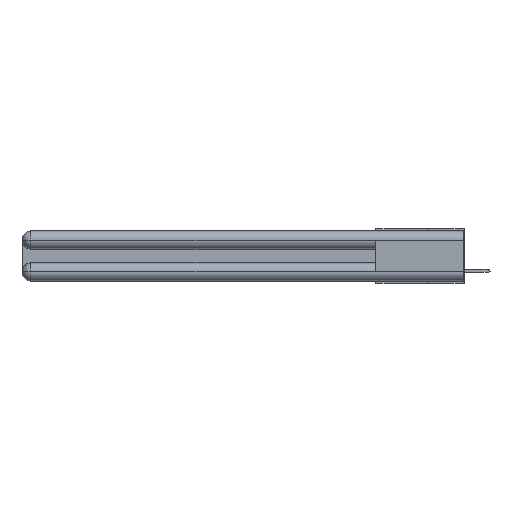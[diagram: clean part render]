
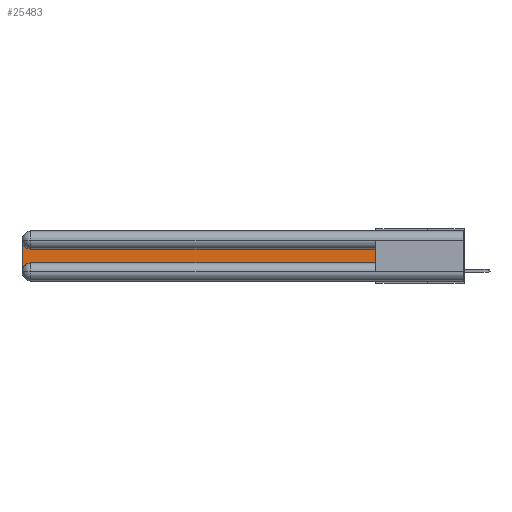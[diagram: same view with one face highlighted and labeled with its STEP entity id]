
A CAD part, left-side view. The second image highlights one B-rep face of the part: STEP entity #25483.
In plain terms, the highlighted planar face has unit normal (-1, 0, 0).
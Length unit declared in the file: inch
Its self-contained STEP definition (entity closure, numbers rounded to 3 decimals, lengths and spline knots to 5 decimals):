
#233 = FACE_OUTER_BOUND ( 'NONE', #18281, .T. ) ;
#754 = ORIENTED_EDGE ( 'NONE', *, *, #1114, .T. ) ;
#1114 = EDGE_CURVE ( 'NONE', #22305, #10074, #21309, .T. ) ;
#3070 = VERTEX_POINT ( 'NONE', #9788 ) ;
#3203 = CARTESIAN_POINT ( 'NONE',  ( 0.075, 3., -0.2175 ) ) ;
#3889 = CARTESIAN_POINT ( 'NONE',  ( 0.075, 0.6, -0.2175 ) ) ;
#4226 = CARTESIAN_POINT ( 'NONE',  ( 0.075, 2.94, -0.2175 ) ) ;
#4910 = ORIENTED_EDGE ( 'NONE', *, *, #23631, .T. ) ;
#5652 = VERTEX_POINT ( 'NONE', #27486 ) ;
#5672 = ORIENTED_EDGE ( 'NONE', *, *, #25782, .T. ) ;
#5896 = CARTESIAN_POINT ( 'NONE',  ( 0.075, 2.94, -0.1225 ) ) ;
#7028 = DIRECTION ( 'NONE',  ( 1., 0., 0. ) ) ;
#7158 = EDGE_CURVE ( 'NONE', #3070, #12762, #14640, .T. ) ;
#8700 = ORIENTED_EDGE ( 'NONE', *, *, #21315, .T. ) ;
#8756 = DIRECTION ( 'NONE',  ( 1., 0., 0. ) ) ;
#9788 = CARTESIAN_POINT ( 'NONE',  ( 0.075, 3., -0.2775 ) ) ;
#9934 = CIRCLE ( 'NONE', #12007, 0.06 ) ;
#10074 = VERTEX_POINT ( 'NONE', #5896 ) ;
#11092 = VECTOR ( 'NONE', #24347, 39.37008 ) ;
#11602 = VECTOR ( 'NONE', #26662, 39.37008 ) ;
#12007 = AXIS2_PLACEMENT_3D ( 'NONE', #19450, #8756, #13043 ) ;
#12559 = VERTEX_POINT ( 'NONE', #3889 ) ;
#12762 = VERTEX_POINT ( 'NONE', #4226 ) ;
#13043 = DIRECTION ( 'NONE',  ( 0., 0., -1. ) ) ;
#13358 = AXIS2_PLACEMENT_3D ( 'NONE', #27663, #16959, #21191 ) ;
#14640 = CIRCLE ( 'NONE', #13358, 0.06 ) ;
#15585 = DIRECTION ( 'NONE',  ( 0., -1., 0. ) ) ;
#15611 = CARTESIAN_POINT ( 'NONE',  ( 0.075, 0.6, -0.2175 ) ) ;
#15992 = DIRECTION ( 'NONE',  ( 0., 0., -1. ) ) ;
#16319 = VECTOR ( 'NONE', #15585, 39.37008 ) ;
#16651 = LINE ( 'NONE', #26380, #16319 ) ;
#16959 = DIRECTION ( 'NONE',  ( 1., 0., 0. ) ) ;
#18281 = EDGE_LOOP ( 'NONE', ( #754, #5672, #8700, #24886, #24670, #4910 ) ) ;
#18318 = CARTESIAN_POINT ( 'NONE',  ( 0.075, 0.6, -0.1225 ) ) ;
#19450 = CARTESIAN_POINT ( 'NONE',  ( 0.075, 2.94, -0.0625 ) ) ;
#19939 = CARTESIAN_POINT ( 'NONE',  ( 0.075, 0.6, -0.1225 ) ) ;
#20335 = LINE ( 'NONE', #3203, #11602 ) ;
#21177 = LINE ( 'NONE', #15611, #11092 ) ;
#21191 = DIRECTION ( 'NONE',  ( 0., 0., -1. ) ) ;
#21201 = EDGE_CURVE ( 'NONE', #12762, #12559, #16651, .T. ) ;
#21309 = LINE ( 'NONE', #18318, #27019 ) ;
#21315 = EDGE_CURVE ( 'NONE', #5652, #3070, #20335, .T. ) ;
#22115 = PLANE ( 'NONE',  #22648 ) ;
#22305 = VERTEX_POINT ( 'NONE', #19939 ) ;
#22648 = AXIS2_PLACEMENT_3D ( 'NONE', #26631, #7028, #15992 ) ;
#23631 = EDGE_CURVE ( 'NONE', #12559, #22305, #21177, .T. ) ;
#23639 = DIRECTION ( 'NONE',  ( 0., 1., 0. ) ) ;
#24347 = DIRECTION ( 'NONE',  ( 0., 0., 1. ) ) ;
#24670 = ORIENTED_EDGE ( 'NONE', *, *, #21201, .T. ) ;
#24886 = ORIENTED_EDGE ( 'NONE', *, *, #7158, .T. ) ;
#25483 = ADVANCED_FACE ( 'NONE', ( #233 ), #22115, .F. ) ;
#25782 = EDGE_CURVE ( 'NONE', #10074, #5652, #9934, .T. ) ;
#26380 = CARTESIAN_POINT ( 'NONE',  ( 0.075, 0.6, -0.2175 ) ) ;
#26631 = CARTESIAN_POINT ( 'NONE',  ( 0.075, 3., -0.1225 ) ) ;
#26662 = DIRECTION ( 'NONE',  ( 0., 0., -1. ) ) ;
#27019 = VECTOR ( 'NONE', #23639, 39.37008 ) ;
#27486 = CARTESIAN_POINT ( 'NONE',  ( 0.075, 3., -0.0625 ) ) ;
#27663 = CARTESIAN_POINT ( 'NONE',  ( 0.075, 2.94, -0.2775 ) ) ;
